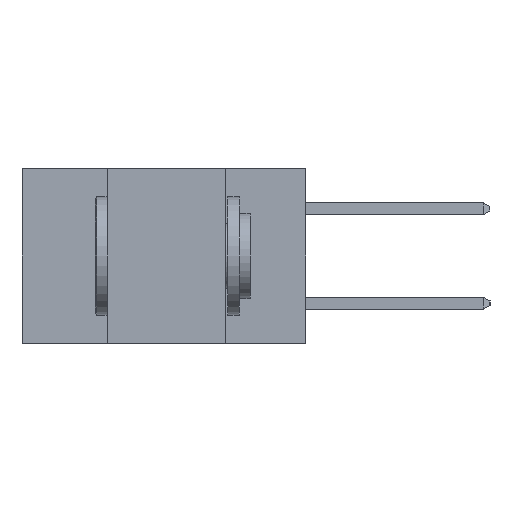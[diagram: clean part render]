
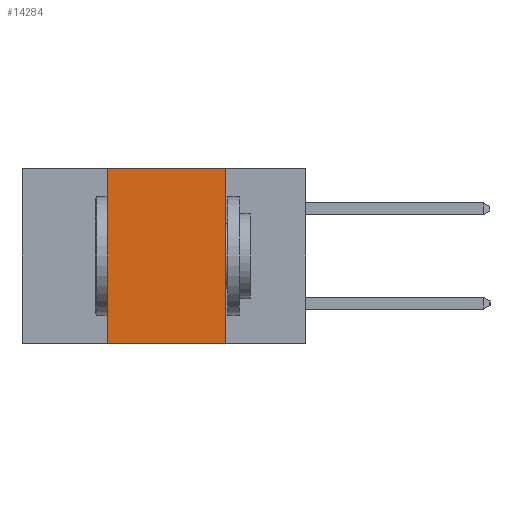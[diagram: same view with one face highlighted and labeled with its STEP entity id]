
A CAD part, left-side view. The second image highlights one B-rep face of the part: STEP entity #14284.
In plain terms, the highlighted planar face has unit normal (-1, 0, 0).
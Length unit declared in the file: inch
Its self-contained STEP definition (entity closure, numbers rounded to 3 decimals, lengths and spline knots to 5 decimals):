
#320 = CARTESIAN_POINT ( 'NONE',  ( 0., 0.42, -0.37 ) ) ;
#697 = PLANE ( 'NONE',  #11291 ) ;
#978 = LINE ( 'NONE', #11004, #11095 ) ;
#1107 = EDGE_CURVE ( 'NONE', #10474, #14275, #978, .T. ) ;
#1677 = DIRECTION ( 'NONE',  ( 0., 0., 1. ) ) ;
#1771 = ORIENTED_EDGE ( 'NONE', *, *, #3983, .F. ) ;
#2341 = EDGE_LOOP ( 'NONE', ( #1771, #9994, #4624, #2581 ) ) ;
#2533 = EDGE_CURVE ( 'NONE', #4082, #14558, #4028, .T. ) ;
#2581 = ORIENTED_EDGE ( 'NONE', *, *, #2533, .T. ) ;
#3196 = VECTOR ( 'NONE', #9226, 39.37008 ) ;
#3341 = DIRECTION ( 'NONE',  ( 0., 0., -1. ) ) ;
#3983 = EDGE_CURVE ( 'NONE', #14275, #14558, #14268, .T. ) ;
#4028 = LINE ( 'NONE', #10725, #3196 ) ;
#4043 = CARTESIAN_POINT ( 'NONE',  ( 0., 0.17, -0.37 ) ) ;
#4082 = VERTEX_POINT ( 'NONE', #7599 ) ;
#4187 = VECTOR ( 'NONE', #6337, 39.37008 ) ;
#4364 = FACE_OUTER_BOUND ( 'NONE', #2341, .T. ) ;
#4624 = ORIENTED_EDGE ( 'NONE', *, *, #13383, .F. ) ;
#6337 = DIRECTION ( 'NONE',  ( 0., 0., -1. ) ) ;
#7599 = CARTESIAN_POINT ( 'NONE',  ( 0., 0.42, -0.37 ) ) ;
#8314 = LINE ( 'NONE', #320, #14895 ) ;
#9226 = DIRECTION ( 'NONE',  ( 0., -1., 0. ) ) ;
#9425 = CARTESIAN_POINT ( 'NONE',  ( 0., 0.17, -0.37 ) ) ;
#9871 = CARTESIAN_POINT ( 'NONE',  ( 0., 0.6, 0. ) ) ;
#9994 = ORIENTED_EDGE ( 'NONE', *, *, #1107, .F. ) ;
#10407 = CARTESIAN_POINT ( 'NONE',  ( 0., 0.42, 0. ) ) ;
#10474 = VERTEX_POINT ( 'NONE', #10407 ) ;
#10725 = CARTESIAN_POINT ( 'NONE',  ( 0., 0.6, -0.37 ) ) ;
#11004 = CARTESIAN_POINT ( 'NONE',  ( 0., 0.6, 0. ) ) ;
#11095 = VECTOR ( 'NONE', #12785, 39.37008 ) ;
#11251 = DIRECTION ( 'NONE',  ( 1., 0., 0. ) ) ;
#11291 = AXIS2_PLACEMENT_3D ( 'NONE', #9871, #11251, #3341 ) ;
#12785 = DIRECTION ( 'NONE',  ( 0., -1., 0. ) ) ;
#13383 = EDGE_CURVE ( 'NONE', #4082, #10474, #8314, .T. ) ;
#14268 = LINE ( 'NONE', #4043, #4187 ) ;
#14275 = VERTEX_POINT ( 'NONE', #16457 ) ;
#14284 = ADVANCED_FACE ( 'NONE', ( #4364 ), #697, .F. ) ;
#14558 = VERTEX_POINT ( 'NONE', #9425 ) ;
#14895 = VECTOR ( 'NONE', #1677, 39.37008 ) ;
#16457 = CARTESIAN_POINT ( 'NONE',  ( 0., 0.17, 0. ) ) ;
